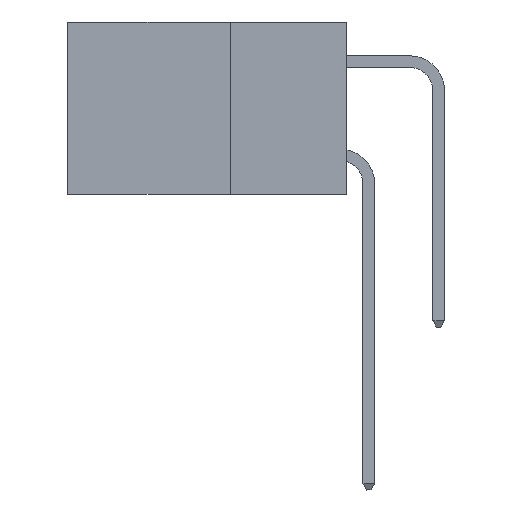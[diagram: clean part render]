
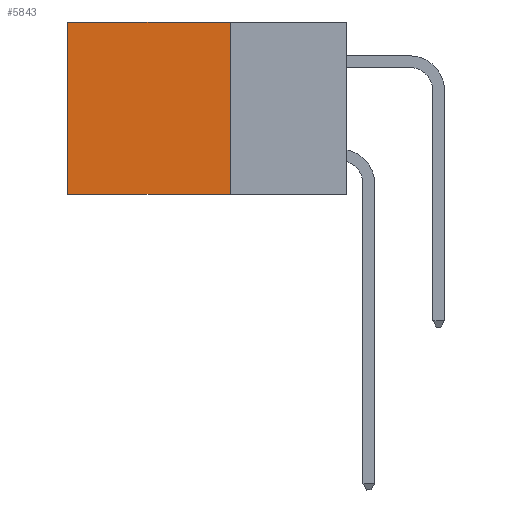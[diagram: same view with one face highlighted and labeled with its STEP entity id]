
A CAD part, left-side view. The second image highlights one B-rep face of the part: STEP entity #5843.
In plain terms, the highlighted planar face has unit normal (-1, 0, 0).
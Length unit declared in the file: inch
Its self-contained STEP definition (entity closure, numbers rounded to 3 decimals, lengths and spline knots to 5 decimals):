
#742 = EDGE_CURVE ( 'NONE', #36954, #23327, #13226, .T. ) ;
#1072 = CARTESIAN_POINT ( 'NONE',  ( 0.2875, 0.25, 0. ) ) ;
#2192 = EDGE_CURVE ( 'NONE', #23327, #38847, #2256, .T. ) ;
#2256 = LINE ( 'NONE', #4309, #7480 ) ;
#4309 = CARTESIAN_POINT ( 'NONE',  ( 0.2875, 0.25, -0.37 ) ) ;
#5843 = ADVANCED_FACE ( 'NONE', ( #32265 ), #12355, .F. ) ;
#6558 = CARTESIAN_POINT ( 'NONE',  ( 0.2875, 0.6, 0. ) ) ;
#7112 = CARTESIAN_POINT ( 'NONE',  ( 0.2875, 0.25, -0.37 ) ) ;
#7225 = DIRECTION ( 'NONE',  ( 0., 0., -1. ) ) ;
#7480 = VECTOR ( 'NONE', #30961, 39.37008 ) ;
#10708 = ORIENTED_EDGE ( 'NONE', *, *, #26018, .T. ) ;
#12223 = VECTOR ( 'NONE', #24907, 39.37008 ) ;
#12355 = PLANE ( 'NONE',  #20100 ) ;
#12944 = EDGE_CURVE ( 'NONE', #36954, #35836, #17148, .T. ) ;
#13132 = DIRECTION ( 'NONE',  ( 1., 0., 0. ) ) ;
#13226 = LINE ( 'NONE', #1072, #14175 ) ;
#14175 = VECTOR ( 'NONE', #25140, 39.37008 ) ;
#14195 = CARTESIAN_POINT ( 'NONE',  ( 0.2875, 0.6, 0. ) ) ;
#14781 = EDGE_LOOP ( 'NONE', ( #10708, #37006, #26572, #37410 ) ) ;
#17148 = LINE ( 'NONE', #33469, #27558 ) ;
#19890 = CARTESIAN_POINT ( 'NONE',  ( 0.2875, 0.6, -0.37 ) ) ;
#20100 = AXIS2_PLACEMENT_3D ( 'NONE', #31239, #13132, #7225 ) ;
#20251 = LINE ( 'NONE', #6558, #12223 ) ;
#23327 = VERTEX_POINT ( 'NONE', #7112 ) ;
#24907 = DIRECTION ( 'NONE',  ( 0., 0., -1. ) ) ;
#25140 = DIRECTION ( 'NONE',  ( 0., 0., -1. ) ) ;
#26018 = EDGE_CURVE ( 'NONE', #35836, #38847, #20251, .T. ) ;
#26572 = ORIENTED_EDGE ( 'NONE', *, *, #742, .F. ) ;
#27558 = VECTOR ( 'NONE', #33847, 39.37008 ) ;
#30961 = DIRECTION ( 'NONE',  ( 0., 1., 0. ) ) ;
#31239 = CARTESIAN_POINT ( 'NONE',  ( 0.2875, 0.25, 0. ) ) ;
#32265 = FACE_OUTER_BOUND ( 'NONE', #14781, .T. ) ;
#33469 = CARTESIAN_POINT ( 'NONE',  ( 0.2875, 0.25, 0. ) ) ;
#33847 = DIRECTION ( 'NONE',  ( 0., 1., 0. ) ) ;
#34365 = CARTESIAN_POINT ( 'NONE',  ( 0.2875, 0.25, 0. ) ) ;
#35836 = VERTEX_POINT ( 'NONE', #14195 ) ;
#36954 = VERTEX_POINT ( 'NONE', #34365 ) ;
#37006 = ORIENTED_EDGE ( 'NONE', *, *, #2192, .F. ) ;
#37410 = ORIENTED_EDGE ( 'NONE', *, *, #12944, .T. ) ;
#38847 = VERTEX_POINT ( 'NONE', #19890 ) ;
